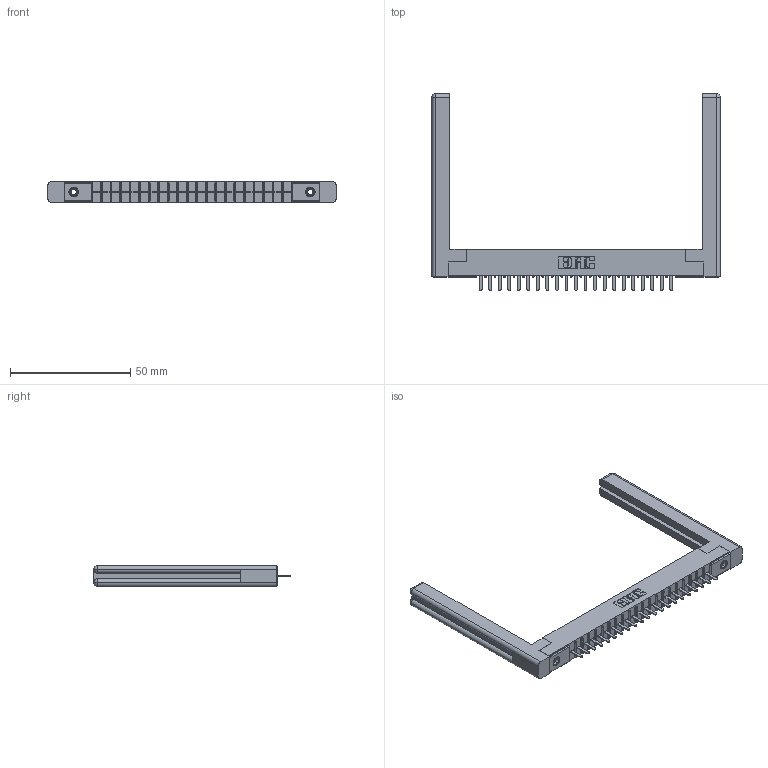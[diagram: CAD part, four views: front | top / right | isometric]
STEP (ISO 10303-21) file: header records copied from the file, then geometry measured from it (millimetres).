
FILE_DESCRIPTION (( 'STEP AP203' ), '1' );
FILE_NAME ('306-021-420-158.STEP', '2020-09-21T20:55:14', ( '' ), ( '' ), 'SwSTEP 2.0', 'SolidWorks 2020', '' );
FILE_SCHEMA (( 'CONFIG_CONTROL_DESIGN' ));
Length unit declared in the file: inch
Products named in the file (5): 306-021-420-158; 345-250-001_345-250-001-102; 306-290-001_120; 306 Part_.156 Dia; 307-220-058
Assembly tree (26 placements, depth 2):
  306-021-420-158
    306 Part_.156 Dia
    306-290-001_120  x21
    345-250-001_345-250-001-102  x2
    307-220-058  x2
Bounding box: 119.84 x 81.76 x 8.71 mm (x, y, z)
Volume: 15836.6 mm3; surface area: 17380.7 mm2
Topology: 26 solids, 26 shells, 1728 faces, 4807 edges, 3078 vertices
Faces by surface type: plane 1139, cylinder 481, sphere 84, cone 12, torus 12
Entity records: 24893 total; most frequent: CARTESIAN_POINT 4185, ORIENTED_EDGE 4088, DIRECTION 4084, EDGE_CURVE 2044, LINE 1582, VECTOR 1582, VERTEX_POINT 1298, AXIS2_PLACEMENT_3D 1251
